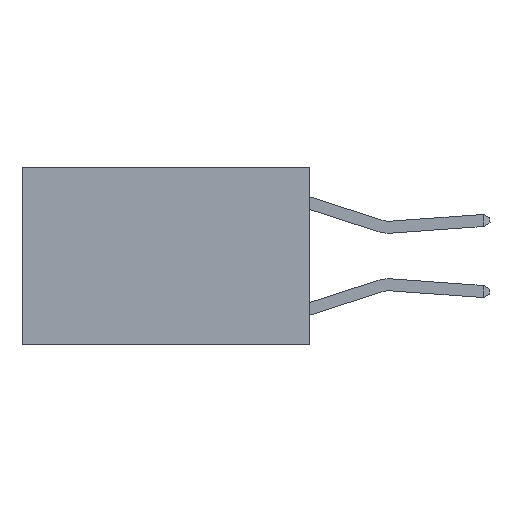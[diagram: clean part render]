
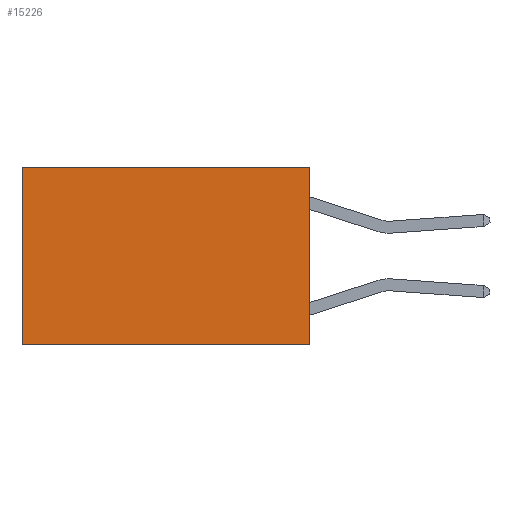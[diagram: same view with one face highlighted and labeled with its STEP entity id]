
A CAD part, left-side view. The second image highlights one B-rep face of the part: STEP entity #15226.
In plain terms, the highlighted planar face has unit normal (-1, 0, 0).
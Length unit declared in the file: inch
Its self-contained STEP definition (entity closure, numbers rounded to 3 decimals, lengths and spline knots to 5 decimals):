
#102 = CARTESIAN_POINT ( 'NONE',  ( 0.2625, 0., -0.37 ) ) ;
#169 = CARTESIAN_POINT ( 'NONE',  ( 0.2625, 0., 0. ) ) ;
#1520 = VECTOR ( 'NONE', #3645, 39.37008 ) ;
#1927 = DIRECTION ( 'NONE',  ( 0., 0., -1. ) ) ;
#2009 = CARTESIAN_POINT ( 'NONE',  ( 0.2625, 0., -0.37 ) ) ;
#2890 = LINE ( 'NONE', #102, #10964 ) ;
#3645 = DIRECTION ( 'NONE',  ( 0., 1., 0. ) ) ;
#4158 = ORIENTED_EDGE ( 'NONE', *, *, #12441, .T. ) ;
#4499 = EDGE_CURVE ( 'NONE', #14026, #5908, #2890, .T. ) ;
#4792 = CARTESIAN_POINT ( 'NONE',  ( 0.2625, 0., 0. ) ) ;
#5311 = DIRECTION ( 'NONE',  ( 0., 1., 0. ) ) ;
#5908 = VERTEX_POINT ( 'NONE', #18368 ) ;
#6542 = DIRECTION ( 'NONE',  ( 0., 0., -1. ) ) ;
#6676 = ORIENTED_EDGE ( 'NONE', *, *, #19346, .T. ) ;
#7057 = PLANE ( 'NONE',  #8881 ) ;
#8143 = LINE ( 'NONE', #4792, #16761 ) ;
#8881 = AXIS2_PLACEMENT_3D ( 'NONE', #169, #12256, #1927 ) ;
#10964 = VECTOR ( 'NONE', #5311, 39.37008 ) ;
#11185 = LINE ( 'NONE', #11489, #19659 ) ;
#11385 = FACE_OUTER_BOUND ( 'NONE', #20326, .T. ) ;
#11489 = CARTESIAN_POINT ( 'NONE',  ( 0.2625, 0.6, 0. ) ) ;
#12250 = CARTESIAN_POINT ( 'NONE',  ( 0.2625, 0., 0. ) ) ;
#12256 = DIRECTION ( 'NONE',  ( 1., 0., 0. ) ) ;
#12441 = EDGE_CURVE ( 'NONE', #21317, #5908, #11185, .T. ) ;
#13227 = DIRECTION ( 'NONE',  ( 0., 0., -1. ) ) ;
#13762 = EDGE_CURVE ( 'NONE', #19516, #14026, #8143, .T. ) ;
#14026 = VERTEX_POINT ( 'NONE', #2009 ) ;
#15226 = ADVANCED_FACE ( 'NONE', ( #11385 ), #7057, .F. ) ;
#15252 = LINE ( 'NONE', #12250, #1520 ) ;
#16761 = VECTOR ( 'NONE', #6542, 39.37008 ) ;
#18368 = CARTESIAN_POINT ( 'NONE',  ( 0.2625, 0.6, -0.37 ) ) ;
#19346 = EDGE_CURVE ( 'NONE', #19516, #21317, #15252, .T. ) ;
#19388 = CARTESIAN_POINT ( 'NONE',  ( 0.2625, 0., 0. ) ) ;
#19516 = VERTEX_POINT ( 'NONE', #19388 ) ;
#19659 = VECTOR ( 'NONE', #13227, 39.37008 ) ;
#20326 = EDGE_LOOP ( 'NONE', ( #4158, #21651, #21175, #6676 ) ) ;
#21175 = ORIENTED_EDGE ( 'NONE', *, *, #13762, .F. ) ;
#21317 = VERTEX_POINT ( 'NONE', #22018 ) ;
#21651 = ORIENTED_EDGE ( 'NONE', *, *, #4499, .F. ) ;
#22018 = CARTESIAN_POINT ( 'NONE',  ( 0.2625, 0.6, 0. ) ) ;
